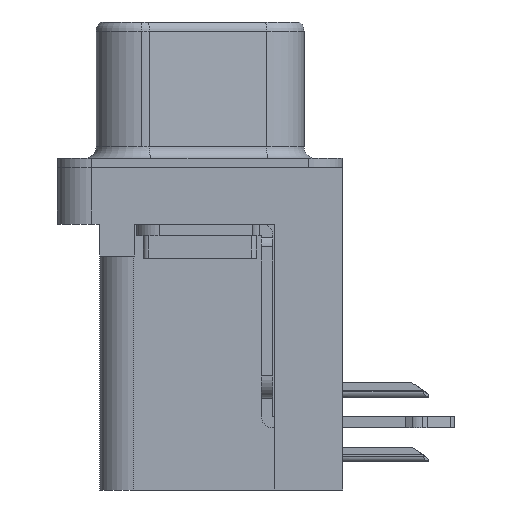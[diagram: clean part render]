
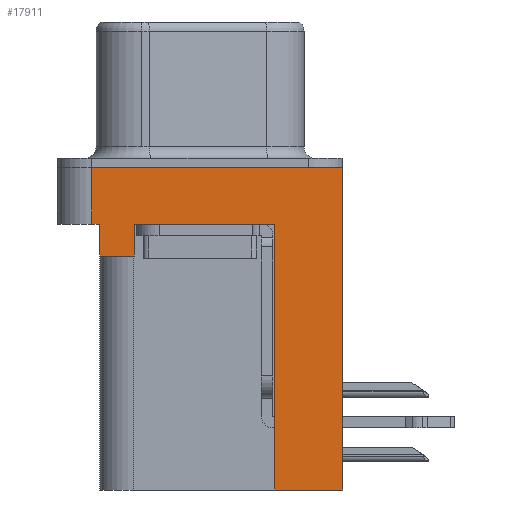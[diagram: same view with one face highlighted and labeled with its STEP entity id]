
A CAD part, left-side view. The second image highlights one B-rep face of the part: STEP entity #17911.
In plain terms, the highlighted planar face has unit normal (-1, 0, 0).
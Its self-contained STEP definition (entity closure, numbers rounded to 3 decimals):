
#434 = CARTESIAN_POINT ( 'NONE',  ( -3., -3.295, -14.2 ) ) ;
#528 = VERTEX_POINT ( 'NONE', #4859 ) ;
#786 = DIRECTION ( 'NONE',  ( 0., -1., 0. ) ) ;
#999 = ORIENTED_EDGE ( 'NONE', *, *, #13024, .F. ) ;
#1367 = VECTOR ( 'NONE', #18952, 1000. ) ;
#1394 = VERTEX_POINT ( 'NONE', #19129 ) ;
#1573 = FACE_OUTER_BOUND ( 'NONE', #19532, .T. ) ;
#1587 = EDGE_CURVE ( 'NONE', #528, #13425, #16455, .T. ) ;
#1947 = DIRECTION ( 'NONE',  ( 0., 0., 1. ) ) ;
#1992 = VERTEX_POINT ( 'NONE', #18127 ) ;
#2374 = ORIENTED_EDGE ( 'NONE', *, *, #1587, .F. ) ;
#2730 = CARTESIAN_POINT ( 'NONE',  ( -3., 4.425, -3.9 ) ) ;
#2850 = ORIENTED_EDGE ( 'NONE', *, *, #6000, .F. ) ;
#3289 = EDGE_CURVE ( 'NONE', #1394, #19395, #18028, .T. ) ;
#3745 = VERTEX_POINT ( 'NONE', #7928 ) ;
#4349 = VERTEX_POINT ( 'NONE', #19026 ) ;
#4400 = CARTESIAN_POINT ( 'NONE',  ( -3., 4.775, 0. ) ) ;
#4859 = CARTESIAN_POINT ( 'NONE',  ( -3., 4.775, -2.5 ) ) ;
#5018 = CARTESIAN_POINT ( 'NONE',  ( -3., 4.775, -2.5 ) ) ;
#5212 = CARTESIAN_POINT ( 'NONE',  ( -3., 2.895, -3.9 ) ) ;
#5262 = DIRECTION ( 'NONE',  ( 0., 0., 1. ) ) ;
#5520 = LINE ( 'NONE', #5212, #6271 ) ;
#5618 = CARTESIAN_POINT ( 'NONE',  ( -3., -6.275, -2.5 ) ) ;
#5859 = VECTOR ( 'NONE', #5262, 1000. ) ;
#6000 = EDGE_CURVE ( 'NONE', #13425, #4349, #13601, .T. ) ;
#6266 = CARTESIAN_POINT ( 'NONE',  ( -3., -3.295, -14.2 ) ) ;
#6271 = VECTOR ( 'NONE', #18040, 1000. ) ;
#6705 = CARTESIAN_POINT ( 'NONE',  ( -3., -6.275, -2.5 ) ) ;
#6779 = DIRECTION ( 'NONE',  ( 0., 1., 0. ) ) ;
#7528 = ORIENTED_EDGE ( 'NONE', *, *, #11194, .T. ) ;
#7812 = LINE ( 'NONE', #2730, #1367 ) ;
#7928 = CARTESIAN_POINT ( 'NONE',  ( -3., 4.425, -3.9 ) ) ;
#9743 = VECTOR ( 'NONE', #1947, 1000. ) ;
#9819 = VECTOR ( 'NONE', #6779, 1000. ) ;
#10068 = ORIENTED_EDGE ( 'NONE', *, *, #16380, .T. ) ;
#10391 = LINE ( 'NONE', #11883, #13081 ) ;
#10796 = ORIENTED_EDGE ( 'NONE', *, *, #20920, .T. ) ;
#10888 = DIRECTION ( 'NONE',  ( -1., 0., 0. ) ) ;
#10977 = CARTESIAN_POINT ( 'NONE',  ( -3., 4.425, -2.5 ) ) ;
#11041 = ORIENTED_EDGE ( 'NONE', *, *, #11153, .F. ) ;
#11153 = EDGE_CURVE ( 'NONE', #3745, #11768, #13579, .T. ) ;
#11163 = LINE ( 'NONE', #6705, #11251 ) ;
#11183 = ORIENTED_EDGE ( 'NONE', *, *, #3289, .F. ) ;
#11194 = EDGE_CURVE ( 'NONE', #17404, #17952, #16981, .T. ) ;
#11251 = VECTOR ( 'NONE', #19679, 1000. ) ;
#11493 = VECTOR ( 'NONE', #786, 1000. ) ;
#11768 = VERTEX_POINT ( 'NONE', #10977 ) ;
#11882 = DIRECTION ( 'NONE',  ( 0., 0., 1. ) ) ;
#11883 = CARTESIAN_POINT ( 'NONE',  ( -3., -6.275, -2.5 ) ) ;
#13024 = EDGE_CURVE ( 'NONE', #1992, #3745, #7812, .T. ) ;
#13081 = VECTOR ( 'NONE', #16872, 1000. ) ;
#13311 = LINE ( 'NONE', #19818, #5859 ) ;
#13425 = VERTEX_POINT ( 'NONE', #4400 ) ;
#13579 = LINE ( 'NONE', #15374, #16549 ) ;
#13601 = LINE ( 'NONE', #17003, #11493 ) ;
#13783 = DIRECTION ( 'NONE',  ( 0., -1., 0. ) ) ;
#15374 = CARTESIAN_POINT ( 'NONE',  ( -3., 4.425, -3.9 ) ) ;
#15528 = ORIENTED_EDGE ( 'NONE', *, *, #17255, .F. ) ;
#15885 = CARTESIAN_POINT ( 'NONE',  ( -3., -6.275, -2.5 ) ) ;
#16380 = EDGE_CURVE ( 'NONE', #1394, #4349, #11163, .T. ) ;
#16455 = LINE ( 'NONE', #5018, #9743 ) ;
#16549 = VECTOR ( 'NONE', #11882, 1000. ) ;
#16600 = CARTESIAN_POINT ( 'NONE',  ( -3., 2.895, -2.5 ) ) ;
#16872 = DIRECTION ( 'NONE',  ( 0., -1., 0. ) ) ;
#16981 = LINE ( 'NONE', #5618, #17563 ) ;
#17003 = CARTESIAN_POINT ( 'NONE',  ( -3., -6.275, 0. ) ) ;
#17255 = EDGE_CURVE ( 'NONE', #19395, #17952, #13311, .T. ) ;
#17404 = VERTEX_POINT ( 'NONE', #16600 ) ;
#17485 = CARTESIAN_POINT ( 'NONE',  ( -3., -3.295, -2.5 ) ) ;
#17563 = VECTOR ( 'NONE', #13783, 1000. ) ;
#17911 = ADVANCED_FACE ( 'NONE', ( #1573 ), #19296, .T. ) ;
#17952 = VERTEX_POINT ( 'NONE', #17485 ) ;
#18028 = LINE ( 'NONE', #434, #9819 ) ;
#18040 = DIRECTION ( 'NONE',  ( 0., 0., 1. ) ) ;
#18127 = CARTESIAN_POINT ( 'NONE',  ( -3., 2.895, -3.9 ) ) ;
#18854 = DIRECTION ( 'NONE',  ( 0., 0., 1. ) ) ;
#18904 = ORIENTED_EDGE ( 'NONE', *, *, #19530, .T. ) ;
#18952 = DIRECTION ( 'NONE',  ( 0., 1., 0. ) ) ;
#19026 = CARTESIAN_POINT ( 'NONE',  ( -3., -6.275, 0. ) ) ;
#19129 = CARTESIAN_POINT ( 'NONE',  ( -3., -6.275, -14.2 ) ) ;
#19296 = PLANE ( 'NONE',  #20457 ) ;
#19395 = VERTEX_POINT ( 'NONE', #6266 ) ;
#19530 = EDGE_CURVE ( 'NONE', #1992, #17404, #5520, .T. ) ;
#19532 = EDGE_LOOP ( 'NONE', ( #2850, #2374, #10796, #11041, #999, #18904, #7528, #15528, #11183, #10068 ) ) ;
#19679 = DIRECTION ( 'NONE',  ( 0., 0., 1. ) ) ;
#19818 = CARTESIAN_POINT ( 'NONE',  ( -3., -3.295, -14.2 ) ) ;
#20457 = AXIS2_PLACEMENT_3D ( 'NONE', #15885, #10888, #18854 ) ;
#20920 = EDGE_CURVE ( 'NONE', #528, #11768, #10391, .T. ) ;
